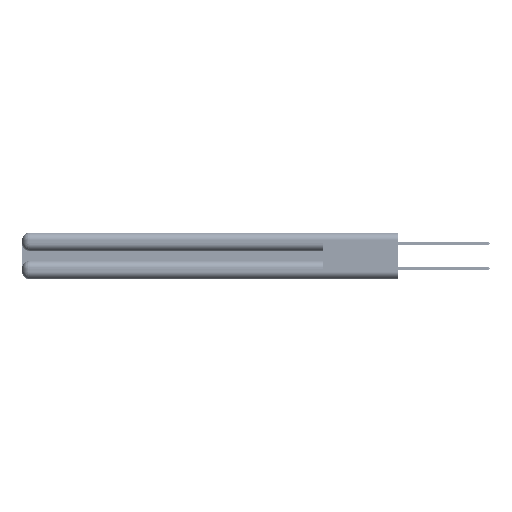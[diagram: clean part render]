
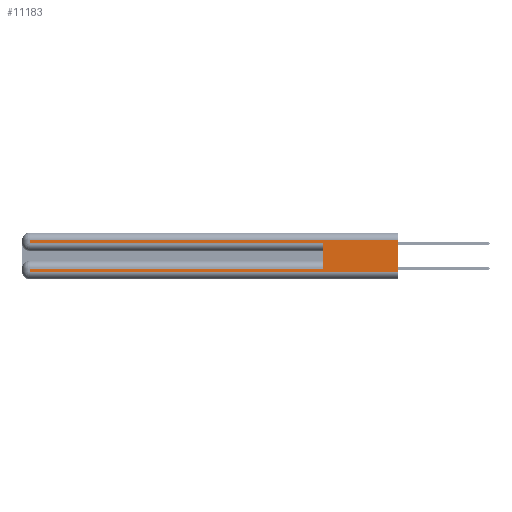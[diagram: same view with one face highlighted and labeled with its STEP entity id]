
A CAD part, left-side view. The second image highlights one B-rep face of the part: STEP entity #11183.
In plain terms, the highlighted planar face has unit normal (-1, 0, 0).
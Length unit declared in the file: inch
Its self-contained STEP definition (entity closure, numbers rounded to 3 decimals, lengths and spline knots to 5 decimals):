
#621 = VERTEX_POINT ( 'NONE', #54767 ) ;
#1061 = VERTEX_POINT ( 'NONE', #26810 ) ;
#1396 = DIRECTION ( 'NONE',  ( 0., 0., 1. ) ) ;
#2454 = VECTOR ( 'NONE', #18486, 39.37008 ) ;
#3952 = ORIENTED_EDGE ( 'NONE', *, *, #21605, .T. ) ;
#4014 = EDGE_CURVE ( 'NONE', #1061, #22377, #24041, .T. ) ;
#4827 = CARTESIAN_POINT ( 'NONE',  ( 0., 0., 0.285 ) ) ;
#5970 = VECTOR ( 'NONE', #21578, 39.37008 ) ;
#6307 = VERTEX_POINT ( 'NONE', #16919 ) ;
#7870 = EDGE_CURVE ( 'NONE', #6307, #19389, #13252, .T. ) ;
#8705 = CARTESIAN_POINT ( 'NONE',  ( 0., 0., 0.06 ) ) ;
#8733 = DIRECTION ( 'NONE',  ( 0., 0., -1. ) ) ;
#9078 = VECTOR ( 'NONE', #23839, 39.37008 ) ;
#9223 = VERTEX_POINT ( 'NONE', #39555 ) ;
#10172 = EDGE_CURVE ( 'NONE', #1061, #9223, #32320, .T. ) ;
#10801 = DIRECTION ( 'NONE',  ( 0., -1., 0. ) ) ;
#11183 = ADVANCED_FACE ( 'NONE', ( #43268 ), #53860, .F. ) ;
#12432 = ORIENTED_EDGE ( 'NONE', *, *, #14950, .T. ) ;
#13252 = LINE ( 'NONE', #35266, #16054 ) ;
#13881 = ORIENTED_EDGE ( 'NONE', *, *, #10172, .T. ) ;
#14649 = CARTESIAN_POINT ( 'NONE',  ( 0., 0.6, 0.145 ) ) ;
#14950 = EDGE_CURVE ( 'NONE', #19389, #22377, #27660, .T. ) ;
#15625 = LINE ( 'NONE', #14649, #19765 ) ;
#16054 = VECTOR ( 'NONE', #43572, 39.37008 ) ;
#16919 = CARTESIAN_POINT ( 'NONE',  ( 0., 2.94, 0.085 ) ) ;
#18486 = DIRECTION ( 'NONE',  ( 0., 1., 0. ) ) ;
#19167 = VERTEX_POINT ( 'NONE', #29313 ) ;
#19389 = VERTEX_POINT ( 'NONE', #21934 ) ;
#19765 = VECTOR ( 'NONE', #1396, 39.37008 ) ;
#20256 = VERTEX_POINT ( 'NONE', #31527 ) ;
#21578 = DIRECTION ( 'NONE',  ( 0., 1., 0. ) ) ;
#21605 = EDGE_CURVE ( 'NONE', #9223, #20256, #45133, .T. ) ;
#21906 = ORIENTED_EDGE ( 'NONE', *, *, #4014, .F. ) ;
#21934 = CARTESIAN_POINT ( 'NONE',  ( 0., 2.94, 0.06 ) ) ;
#22377 = VERTEX_POINT ( 'NONE', #8705 ) ;
#23839 = DIRECTION ( 'NONE',  ( 0., 0., -1. ) ) ;
#23957 = LINE ( 'NONE', #40554, #2454 ) ;
#24041 = LINE ( 'NONE', #52858, #34459 ) ;
#26264 = DIRECTION ( 'NONE',  ( 0., 0., -1. ) ) ;
#26810 = CARTESIAN_POINT ( 'NONE',  ( 0., 0., 0.31 ) ) ;
#27061 = EDGE_CURVE ( 'NONE', #621, #6307, #23957, .T. ) ;
#27281 = CARTESIAN_POINT ( 'NONE',  ( 0., 0., 0.37 ) ) ;
#27660 = LINE ( 'NONE', #32651, #38728 ) ;
#29313 = CARTESIAN_POINT ( 'NONE',  ( 0., 0.6, 0.285 ) ) ;
#30189 = EDGE_LOOP ( 'NONE', ( #21906, #13881, #3952, #39240, #55526, #34206, #57064, #12432 ) ) ;
#30294 = CARTESIAN_POINT ( 'NONE',  ( 0., 0., 0.31 ) ) ;
#31527 = CARTESIAN_POINT ( 'NONE',  ( 0., 2.94, 0.285 ) ) ;
#32320 = LINE ( 'NONE', #30294, #5970 ) ;
#32651 = CARTESIAN_POINT ( 'NONE',  ( 0., 0., 0.06 ) ) ;
#33269 = EDGE_CURVE ( 'NONE', #20256, #19167, #34899, .T. ) ;
#34206 = ORIENTED_EDGE ( 'NONE', *, *, #27061, .T. ) ;
#34459 = VECTOR ( 'NONE', #26264, 39.37008 ) ;
#34899 = LINE ( 'NONE', #4827, #45997 ) ;
#35266 = CARTESIAN_POINT ( 'NONE',  ( 0., 2.94, 0.37 ) ) ;
#35276 = DIRECTION ( 'NONE',  ( 1., 0., 0. ) ) ;
#38728 = VECTOR ( 'NONE', #10801, 39.37008 ) ;
#39240 = ORIENTED_EDGE ( 'NONE', *, *, #33269, .T. ) ;
#39555 = CARTESIAN_POINT ( 'NONE',  ( 0., 2.94, 0.31 ) ) ;
#40554 = CARTESIAN_POINT ( 'NONE',  ( 0., 0., 0.085 ) ) ;
#43268 = FACE_OUTER_BOUND ( 'NONE', #30189, .T. ) ;
#43572 = DIRECTION ( 'NONE',  ( 0., 0., -1. ) ) ;
#44694 = AXIS2_PLACEMENT_3D ( 'NONE', #27281, #35276, #8733 ) ;
#45133 = LINE ( 'NONE', #45916, #9078 ) ;
#45916 = CARTESIAN_POINT ( 'NONE',  ( 0., 2.94, 0.37 ) ) ;
#45997 = VECTOR ( 'NONE', #53483, 39.37008 ) ;
#52858 = CARTESIAN_POINT ( 'NONE',  ( 0., 0., 0.37 ) ) ;
#53483 = DIRECTION ( 'NONE',  ( 0., -1., 0. ) ) ;
#53860 = PLANE ( 'NONE',  #44694 ) ;
#54731 = EDGE_CURVE ( 'NONE', #621, #19167, #15625, .T. ) ;
#54767 = CARTESIAN_POINT ( 'NONE',  ( 0., 0.6, 0.085 ) ) ;
#55526 = ORIENTED_EDGE ( 'NONE', *, *, #54731, .F. ) ;
#57064 = ORIENTED_EDGE ( 'NONE', *, *, #7870, .T. ) ;
